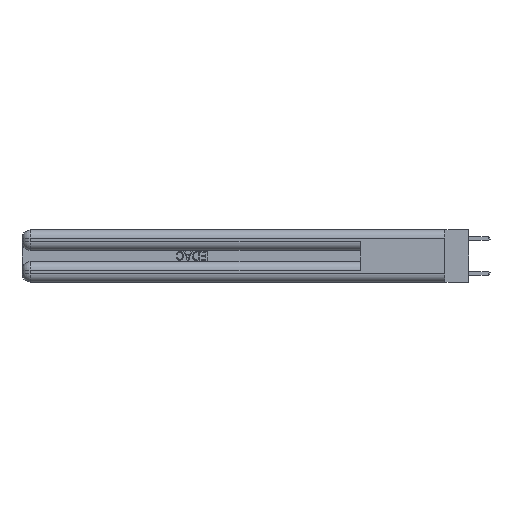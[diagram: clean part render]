
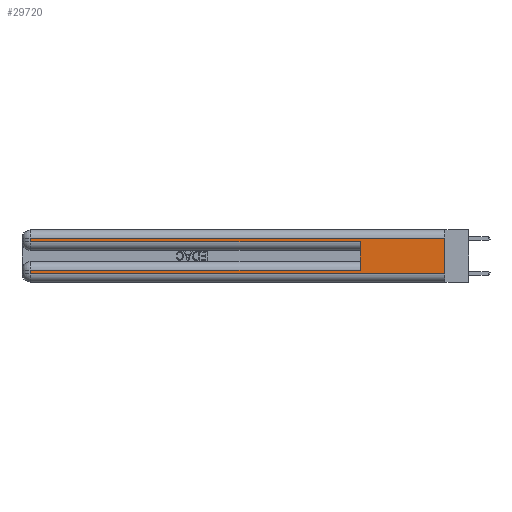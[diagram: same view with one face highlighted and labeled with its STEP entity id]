
A CAD part, left-side view. The second image highlights one B-rep face of the part: STEP entity #29720.
In plain terms, the highlighted planar face has unit normal (-1, 0, 0).
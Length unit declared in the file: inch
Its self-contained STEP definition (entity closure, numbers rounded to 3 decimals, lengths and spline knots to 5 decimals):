
#428 = VECTOR ( 'NONE', #12901, 39.37008 ) ;
#919 = EDGE_LOOP ( 'NONE', ( #20402, #13281, #35754, #10819, #32546, #30121, #18268, #24176 ) ) ;
#1060 = VECTOR ( 'NONE', #16516, 39.37008 ) ;
#1389 = CARTESIAN_POINT ( 'NONE',  ( 0., 0.6, 0.285 ) ) ;
#2181 = CARTESIAN_POINT ( 'NONE',  ( 0., 2.94, 0.06 ) ) ;
#2639 = EDGE_CURVE ( 'NONE', #8000, #32267, #26146, .T. ) ;
#2730 = EDGE_CURVE ( 'NONE', #15941, #23566, #29864, .T. ) ;
#2758 = EDGE_CURVE ( 'NONE', #24411, #23494, #35276, .T. ) ;
#3788 = CARTESIAN_POINT ( 'NONE',  ( 0., 2.94, 0.085 ) ) ;
#3898 = CARTESIAN_POINT ( 'NONE',  ( 0., 0.6, 0.145 ) ) ;
#4416 = EDGE_CURVE ( 'NONE', #24411, #11113, #12150, .T. ) ;
#5138 = CARTESIAN_POINT ( 'NONE',  ( 0., 0., 0.06 ) ) ;
#5477 = CARTESIAN_POINT ( 'NONE',  ( 0., 0., 0.285 ) ) ;
#7540 = VECTOR ( 'NONE', #29311, 39.37008 ) ;
#8000 = VERTEX_POINT ( 'NONE', #11003 ) ;
#8267 = EDGE_CURVE ( 'NONE', #15941, #32267, #15281, .T. ) ;
#9562 = DIRECTION ( 'NONE',  ( 0., 1., 0. ) ) ;
#9790 = CARTESIAN_POINT ( 'NONE',  ( 0., 2.94, 0.37 ) ) ;
#10603 = DIRECTION ( 'NONE',  ( 0., 0., -1. ) ) ;
#10819 = ORIENTED_EDGE ( 'NONE', *, *, #2639, .T. ) ;
#11003 = CARTESIAN_POINT ( 'NONE',  ( 0., 2.94, 0.285 ) ) ;
#11021 = VECTOR ( 'NONE', #12784, 39.37008 ) ;
#11113 = VERTEX_POINT ( 'NONE', #26747 ) ;
#11916 = CARTESIAN_POINT ( 'NONE',  ( 0., 0., 0.31 ) ) ;
#12150 = LINE ( 'NONE', #12512, #428 ) ;
#12182 = CARTESIAN_POINT ( 'NONE',  ( 0., 0., 0.085 ) ) ;
#12363 = VECTOR ( 'NONE', #22923, 39.37008 ) ;
#12512 = CARTESIAN_POINT ( 'NONE',  ( 0., 0., 0.37 ) ) ;
#12657 = AXIS2_PLACEMENT_3D ( 'NONE', #36496, #36124, #10603 ) ;
#12784 = DIRECTION ( 'NONE',  ( 0., 0., -1. ) ) ;
#12901 = DIRECTION ( 'NONE',  ( 0., 0., -1. ) ) ;
#13101 = LINE ( 'NONE', #33202, #27167 ) ;
#13281 = ORIENTED_EDGE ( 'NONE', *, *, #2758, .T. ) ;
#15281 = LINE ( 'NONE', #3898, #12363 ) ;
#15941 = VERTEX_POINT ( 'NONE', #19791 ) ;
#16516 = DIRECTION ( 'NONE',  ( 0., -1., 0. ) ) ;
#17632 = VECTOR ( 'NONE', #22996, 39.37008 ) ;
#18030 = VERTEX_POINT ( 'NONE', #2181 ) ;
#18268 = ORIENTED_EDGE ( 'NONE', *, *, #32269, .T. ) ;
#18627 = EDGE_CURVE ( 'NONE', #18030, #11113, #30663, .T. ) ;
#19791 = CARTESIAN_POINT ( 'NONE',  ( 0., 0.6, 0.085 ) ) ;
#20402 = ORIENTED_EDGE ( 'NONE', *, *, #4416, .F. ) ;
#22388 = LINE ( 'NONE', #9790, #11021 ) ;
#22923 = DIRECTION ( 'NONE',  ( 0., 0., 1. ) ) ;
#22996 = DIRECTION ( 'NONE',  ( 0., -1., 0. ) ) ;
#23494 = VERTEX_POINT ( 'NONE', #32103 ) ;
#23566 = VERTEX_POINT ( 'NONE', #3788 ) ;
#24176 = ORIENTED_EDGE ( 'NONE', *, *, #18627, .T. ) ;
#24411 = VERTEX_POINT ( 'NONE', #11916 ) ;
#24463 = DIRECTION ( 'NONE',  ( 0., 0., -1. ) ) ;
#25128 = PLANE ( 'NONE',  #12657 ) ;
#26146 = LINE ( 'NONE', #5477, #17632 ) ;
#26747 = CARTESIAN_POINT ( 'NONE',  ( 0., 0., 0.06 ) ) ;
#27167 = VECTOR ( 'NONE', #24463, 39.37008 ) ;
#29311 = DIRECTION ( 'NONE',  ( 0., 1., 0. ) ) ;
#29498 = CARTESIAN_POINT ( 'NONE',  ( 0., 0., 0.31 ) ) ;
#29720 = ADVANCED_FACE ( 'NONE', ( #33873 ), #25128, .F. ) ;
#29864 = LINE ( 'NONE', #12182, #33116 ) ;
#30121 = ORIENTED_EDGE ( 'NONE', *, *, #2730, .T. ) ;
#30663 = LINE ( 'NONE', #5138, #1060 ) ;
#32103 = CARTESIAN_POINT ( 'NONE',  ( 0., 2.94, 0.31 ) ) ;
#32267 = VERTEX_POINT ( 'NONE', #1389 ) ;
#32269 = EDGE_CURVE ( 'NONE', #23566, #18030, #22388, .T. ) ;
#32546 = ORIENTED_EDGE ( 'NONE', *, *, #8267, .F. ) ;
#33116 = VECTOR ( 'NONE', #9562, 39.37008 ) ;
#33202 = CARTESIAN_POINT ( 'NONE',  ( 0., 2.94, 0.37 ) ) ;
#33873 = FACE_OUTER_BOUND ( 'NONE', #919, .T. ) ;
#33952 = EDGE_CURVE ( 'NONE', #23494, #8000, #13101, .T. ) ;
#35276 = LINE ( 'NONE', #29498, #7540 ) ;
#35754 = ORIENTED_EDGE ( 'NONE', *, *, #33952, .T. ) ;
#36124 = DIRECTION ( 'NONE',  ( 1., 0., 0. ) ) ;
#36496 = CARTESIAN_POINT ( 'NONE',  ( 0., 0., 0.37 ) ) ;
